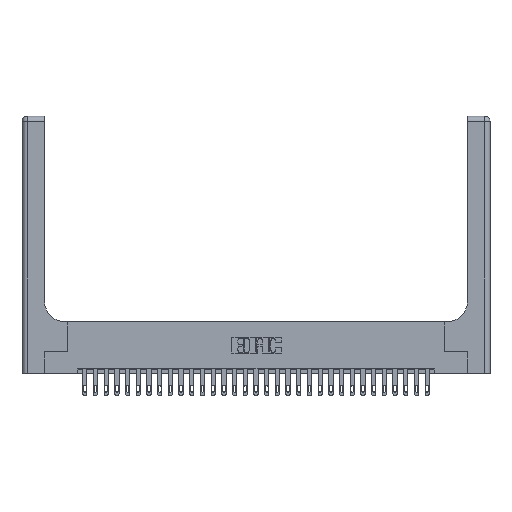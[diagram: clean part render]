
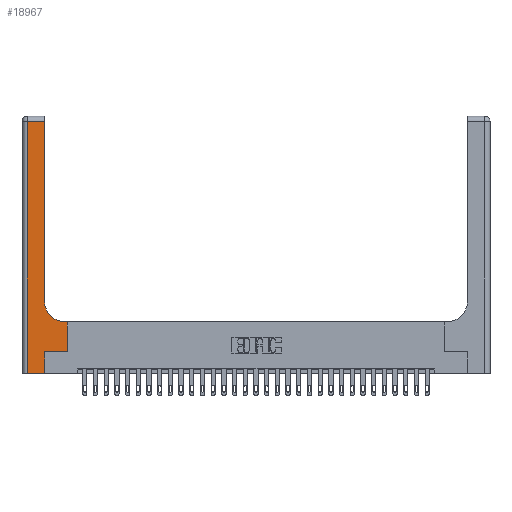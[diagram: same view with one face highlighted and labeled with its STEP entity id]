
A CAD part, top view. The second image highlights one B-rep face of the part: STEP entity #18967.
In plain terms, the highlighted planar face has unit normal (0, 0, 1).
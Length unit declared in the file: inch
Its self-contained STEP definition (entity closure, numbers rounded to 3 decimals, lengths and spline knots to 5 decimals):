
#58 = EDGE_CURVE ( 'NONE', #25306, #1472, #73, .T. ) ;
#73 = LINE ( 'NONE', #11397, #13552 ) ;
#354 = DIRECTION ( 'NONE',  ( -1., 0., 0. ) ) ;
#945 = VECTOR ( 'NONE', #4985, 39.37008 ) ;
#1129 = CIRCLE ( 'NONE', #11217, 0.25 ) ;
#1472 = VERTEX_POINT ( 'NONE', #1761 ) ;
#1761 = CARTESIAN_POINT ( 'NONE',  ( 0.06, 2.94, 0.37 ) ) ;
#1926 = DIRECTION ( 'NONE',  ( 0., 1., 0. ) ) ;
#2299 = EDGE_CURVE ( 'NONE', #9555, #27283, #1129, .T. ) ;
#2870 = CARTESIAN_POINT ( 'NONE',  ( 0., 0., 0.37 ) ) ;
#2884 = ORIENTED_EDGE ( 'NONE', *, *, #16594, .T. ) ;
#3373 = ORIENTED_EDGE ( 'NONE', *, *, #6127, .T. ) ;
#3576 = CARTESIAN_POINT ( 'NONE',  ( 0.51, 0.85, 0.37 ) ) ;
#3577 = EDGE_CURVE ( 'NONE', #1472, #24774, #3886, .T. ) ;
#3886 = LINE ( 'NONE', #19506, #13298 ) ;
#4250 = CARTESIAN_POINT ( 'NONE',  ( 0.51, 0.6, 0.37 ) ) ;
#4383 = LINE ( 'NONE', #6956, #22457 ) ;
#4837 = CARTESIAN_POINT ( 'NONE',  ( 0.26, 0.6, 0.37 ) ) ;
#4985 = DIRECTION ( 'NONE',  ( -1., 0., 0. ) ) ;
#5040 = FACE_OUTER_BOUND ( 'NONE', #5443, .T. ) ;
#5443 = EDGE_LOOP ( 'NONE', ( #2884, #10154, #18808, #21692, #3373, #15689, #27462, #11888, #27404 ) ) ;
#6127 = EDGE_CURVE ( 'NONE', #10924, #21604, #4383, .T. ) ;
#6390 = EDGE_CURVE ( 'NONE', #21604, #21851, #27997, .T. ) ;
#6401 = DIRECTION ( 'NONE',  ( 0., 1., 0. ) ) ;
#6563 = VECTOR ( 'NONE', #1926, 39.37008 ) ;
#6956 = CARTESIAN_POINT ( 'NONE',  ( 0.265, 0., 0.37 ) ) ;
#7051 = DIRECTION ( 'NONE',  ( 0., 0., -1. ) ) ;
#7660 = VECTOR ( 'NONE', #17926, 39.37008 ) ;
#9555 = VERTEX_POINT ( 'NONE', #4250 ) ;
#10154 = ORIENTED_EDGE ( 'NONE', *, *, #58, .T. ) ;
#10924 = VERTEX_POINT ( 'NONE', #21458 ) ;
#11217 = AXIS2_PLACEMENT_3D ( 'NONE', #3576, #25616, #23185 ) ;
#11397 = CARTESIAN_POINT ( 'NONE',  ( 0., 2.94, 0.37 ) ) ;
#11888 = ORIENTED_EDGE ( 'NONE', *, *, #12453, .T. ) ;
#12453 = EDGE_CURVE ( 'NONE', #16520, #9555, #15742, .T. ) ;
#13298 = VECTOR ( 'NONE', #25934, 39.37008 ) ;
#13552 = VECTOR ( 'NONE', #354, 39.37008 ) ;
#14694 = CARTESIAN_POINT ( 'NONE',  ( 0.265, 0.25, 0.37 ) ) ;
#14856 = LINE ( 'NONE', #20780, #6563 ) ;
#15176 = VECTOR ( 'NONE', #23696, 39.37008 ) ;
#15689 = ORIENTED_EDGE ( 'NONE', *, *, #6390, .T. ) ;
#15705 = DIRECTION ( 'NONE',  ( 0., 1., 0. ) ) ;
#15742 = LINE ( 'NONE', #4837, #945 ) ;
#16371 = CARTESIAN_POINT ( 'NONE',  ( 0.265, 0.25, 0.37 ) ) ;
#16520 = VERTEX_POINT ( 'NONE', #22877 ) ;
#16594 = EDGE_CURVE ( 'NONE', #27283, #25306, #24004, .T. ) ;
#17465 = CARTESIAN_POINT ( 'NONE',  ( 0.528, 0.25, 0.37 ) ) ;
#17926 = DIRECTION ( 'NONE',  ( 1., 0., 0. ) ) ;
#18074 = LINE ( 'NONE', #2870, #7660 ) ;
#18651 = CARTESIAN_POINT ( 'NONE',  ( 0.26, 0.85, 0.37 ) ) ;
#18808 = ORIENTED_EDGE ( 'NONE', *, *, #3577, .T. ) ;
#18967 = ADVANCED_FACE ( 'NONE', ( #5040 ), #20388, .F. ) ;
#19506 = CARTESIAN_POINT ( 'NONE',  ( 0.06, 3., 0.37 ) ) ;
#19729 = CARTESIAN_POINT ( 'NONE',  ( 0.26, 3., 0.37 ) ) ;
#19961 = CARTESIAN_POINT ( 'NONE',  ( 0., 3., 0.37 ) ) ;
#20121 = EDGE_CURVE ( 'NONE', #24774, #10924, #18074, .T. ) ;
#20242 = DIRECTION ( 'NONE',  ( -1., 0., 0. ) ) ;
#20388 = PLANE ( 'NONE',  #24575 ) ;
#20780 = CARTESIAN_POINT ( 'NONE',  ( 0.528, 0.25, 0.37 ) ) ;
#21458 = CARTESIAN_POINT ( 'NONE',  ( 0.265, 0., 0.37 ) ) ;
#21604 = VERTEX_POINT ( 'NONE', #16371 ) ;
#21692 = ORIENTED_EDGE ( 'NONE', *, *, #20121, .T. ) ;
#21851 = VERTEX_POINT ( 'NONE', #17465 ) ;
#22457 = VECTOR ( 'NONE', #15705, 39.37008 ) ;
#22877 = CARTESIAN_POINT ( 'NONE',  ( 0.528, 0.6, 0.37 ) ) ;
#23185 = DIRECTION ( 'NONE',  ( 1., 0., 0. ) ) ;
#23577 = VECTOR ( 'NONE', #6401, 39.37008 ) ;
#23696 = DIRECTION ( 'NONE',  ( 1., 0., 0. ) ) ;
#24004 = LINE ( 'NONE', #19729, #23577 ) ;
#24575 = AXIS2_PLACEMENT_3D ( 'NONE', #19961, #7051, #20242 ) ;
#24667 = EDGE_CURVE ( 'NONE', #21851, #16520, #14856, .T. ) ;
#24774 = VERTEX_POINT ( 'NONE', #28019 ) ;
#24974 = CARTESIAN_POINT ( 'NONE',  ( 0.26, 2.94, 0.37 ) ) ;
#25306 = VERTEX_POINT ( 'NONE', #24974 ) ;
#25616 = DIRECTION ( 'NONE',  ( 0., 0., -1. ) ) ;
#25934 = DIRECTION ( 'NONE',  ( 0., -1., 0. ) ) ;
#27283 = VERTEX_POINT ( 'NONE', #18651 ) ;
#27404 = ORIENTED_EDGE ( 'NONE', *, *, #2299, .T. ) ;
#27462 = ORIENTED_EDGE ( 'NONE', *, *, #24667, .T. ) ;
#27997 = LINE ( 'NONE', #14694, #15176 ) ;
#28019 = CARTESIAN_POINT ( 'NONE',  ( 0.06, 0., 0.37 ) ) ;
